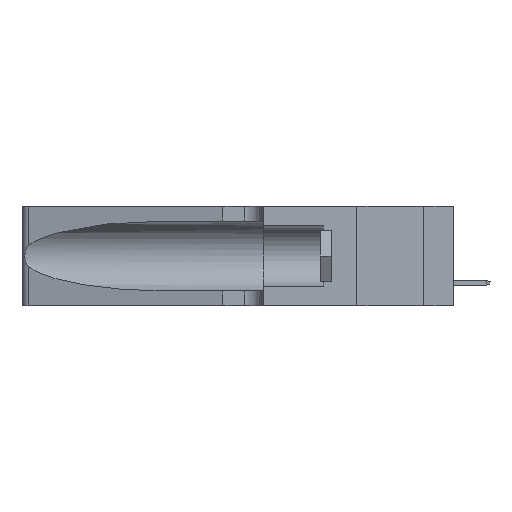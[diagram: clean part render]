
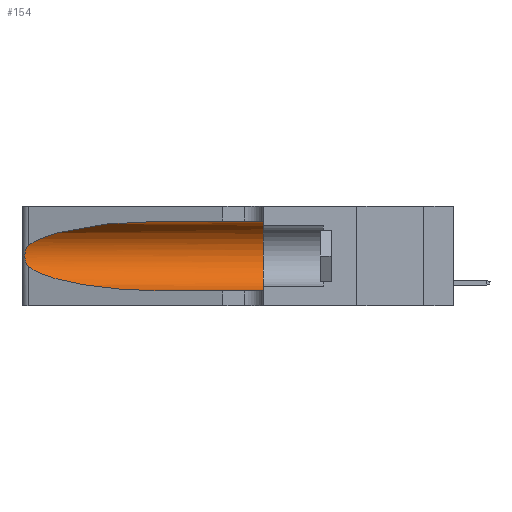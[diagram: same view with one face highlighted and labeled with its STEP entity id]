
A CAD part, left-side view. The second image highlights one B-rep face of the part: STEP entity #154.
In plain terms, the highlighted cylindrical face has radius 3.308 mm (diameter 6.617 mm), a partial arc.
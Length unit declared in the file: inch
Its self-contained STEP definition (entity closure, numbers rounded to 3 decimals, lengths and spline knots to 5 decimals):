
#131 = DIRECTION ( 'NONE',  ( 0., -1., 0. ) ) ;
#154 = ADVANCED_FACE ( 'NONE', ( #12733 ), #5379, .F. ) ;
#813 = ORIENTED_EDGE ( 'NONE', *, *, #28861, .T. ) ;
#963 = CARTESIAN_POINT ( 'NONE',  ( 0.25487, 1.22718, 0.14631 ) ) ;
#1753 = ORIENTED_EDGE ( 'NONE', *, *, #10633, .T. ) ;
#2669 = DIRECTION ( 'NONE',  ( 0., 0., 1. ) ) ;
#2769 = ORIENTED_EDGE ( 'NONE', *, *, #18886, .F. ) ;
#2884 = DIRECTION ( 'NONE',  ( 0., -1., 0. ) ) ;
#3205 = CARTESIAN_POINT ( 'NONE',  ( 0.25787, 1.23484, 0.2124 ) ) ;
#3506 = CARTESIAN_POINT ( 'NONE',  ( 0.25487, 1.22718, 0.22369 ) ) ;
#3818 = EDGE_CURVE ( 'NONE', #5532, #31102, #15495, .T. ) ;
#3832 = CARTESIAN_POINT ( 'NONE',  ( 0.25639, 1.23184, 0.21858 ) ) ;
#3978 = VERTEX_POINT ( 'NONE', #15798 ) ;
#4153 = VERTEX_POINT ( 'NONE', #15297 ) ;
#5379 = CYLINDRICAL_SURFACE ( 'NONE', #9538, 0.13025 ) ;
#5532 = VERTEX_POINT ( 'NONE', #25018 ) ;
#5560 = ORIENTED_EDGE ( 'NONE', *, *, #3818, .T. ) ;
#7277 = EDGE_CURVE ( 'NONE', #7630, #31102, #11832, .T. ) ;
#7630 = VERTEX_POINT ( 'NONE', #8875 ) ;
#8875 = CARTESIAN_POINT ( 'NONE',  ( 0.1305, 0.35, 0.31525 ) ) ;
#9178 = CARTESIAN_POINT ( 'NONE',  ( 0.1305, 0.72297, 0.31525 ) ) ;
#9538 = AXIS2_PLACEMENT_3D ( 'NONE', #10333, #131, #25272 ) ;
#9834 = CARTESIAN_POINT ( 'NONE',  ( 0.1305, 0.35, 0.05475 ) ) ;
#10003 =( BOUNDED_CURVE ( )  B_SPLINE_CURVE ( 3, ( #9178, #18931, #23084, #10980 ),
 .UNSPECIFIED., .F., .F. ) 
 B_SPLINE_CURVE_WITH_KNOTS ( ( 4, 4 ),
 ( 1.5708, 2.84003 ),
 .UNSPECIFIED. ) 
 CURVE ( )  GEOMETRIC_REPRESENTATION_ITEM ( )  RATIONAL_B_SPLINE_CURVE ( ( 1., 0.87, 0.87, 1. ) ) 
 REPRESENTATION_ITEM ( '' )  );
#10169 = CARTESIAN_POINT ( 'NONE',  ( 0.1305, 0.35, 0.185 ) ) ;
#10333 = CARTESIAN_POINT ( 'NONE',  ( 0.1305, 1.61858, 0.185 ) ) ;
#10548 = CARTESIAN_POINT ( 'NONE',  ( 0.26018, 1.23835, 0.19895 ) ) ;
#10633 = EDGE_CURVE ( 'NONE', #3978, #4153, #10003, .T. ) ;
#10980 = CARTESIAN_POINT ( 'NONE',  ( 0.25487, 1.22718, 0.22369 ) ) ;
#11832 = CIRCLE ( 'NONE', #26091, 0.13025 ) ;
#11880 =( BOUNDED_CURVE ( )  B_SPLINE_CURVE ( 3, ( #16994, #21289, #14752, #31005 ),
 .UNSPECIFIED., .F., .F. ) 
 B_SPLINE_CURVE_WITH_KNOTS ( ( 4, 4 ),
 ( 3.44316, 4.71239 ),
 .UNSPECIFIED. ) 
 CURVE ( )  GEOMETRIC_REPRESENTATION_ITEM ( )  RATIONAL_B_SPLINE_CURVE ( ( 1., 0.87, 0.87, 1. ) ) 
 REPRESENTATION_ITEM ( '' )  );
#12733 = FACE_OUTER_BOUND ( 'NONE', #21869, .T. ) ;
#14416 = CARTESIAN_POINT ( 'NONE',  ( 0.1305, 1.61858, 0.31525 ) ) ;
#14752 = CARTESIAN_POINT ( 'NONE',  ( 0.18966, 0.96281, 0.05475 ) ) ;
#15004 = VERTEX_POINT ( 'NONE', #24596 ) ;
#15297 = CARTESIAN_POINT ( 'NONE',  ( 0.25487, 1.22718, 0.22369 ) ) ;
#15495 = LINE ( 'NONE', #25210, #24383 ) ;
#15648 = CARTESIAN_POINT ( 'NONE',  ( 0.26075, 1.23896, 0.19203 ) ) ;
#15798 = CARTESIAN_POINT ( 'NONE',  ( 0.1305, 0.72297, 0.31525 ) ) ;
#15803 = EDGE_CURVE ( 'NONE', #15004, #5532, #11880, .T. ) ;
#16994 = CARTESIAN_POINT ( 'NONE',  ( 0.25487, 1.22718, 0.14631 ) ) ;
#18886 = EDGE_CURVE ( 'NONE', #3978, #7630, #26689, .T. ) ;
#18931 = CARTESIAN_POINT ( 'NONE',  ( 0.18966, 0.96281, 0.31525 ) ) ;
#20416 = CARTESIAN_POINT ( 'NONE',  ( 0.25639, 1.23186, 0.15144 ) ) ;
#20584 = CARTESIAN_POINT ( 'NONE',  ( 0.26075, 1.23896, 0.178 ) ) ;
#21111 = ORIENTED_EDGE ( 'NONE', *, *, #7277, .F. ) ;
#21289 = CARTESIAN_POINT ( 'NONE',  ( 0.2373, 1.15595, 0.08982 ) ) ;
#21517 = ORIENTED_EDGE ( 'NONE', *, *, #15803, .T. ) ;
#21869 = EDGE_LOOP ( 'NONE', ( #1753, #813, #21517, #5560, #21111, #2769 ) ) ;
#22811 = CARTESIAN_POINT ( 'NONE',  ( 0.25854, 1.2359, 0.20912 ) ) ;
#22967 = CARTESIAN_POINT ( 'NONE',  ( 0.25555, 1.22994, 0.2215 ) ) ;
#23084 = CARTESIAN_POINT ( 'NONE',  ( 0.2373, 1.15595, 0.28018 ) ) ;
#24383 = VECTOR ( 'NONE', #2884, 39.37008 ) ;
#24596 = CARTESIAN_POINT ( 'NONE',  ( 0.25487, 1.22718, 0.14631 ) ) ;
#25018 = CARTESIAN_POINT ( 'NONE',  ( 0.1305, 0.72297, 0.05475 ) ) ;
#25056 = CARTESIAN_POINT ( 'NONE',  ( 0.26017, 1.23833, 0.17102 ) ) ;
#25210 = CARTESIAN_POINT ( 'NONE',  ( 0.1305, 1.61858, 0.05475 ) ) ;
#25272 = DIRECTION ( 'NONE',  ( 0., 0., -1. ) ) ;
#25360 = CARTESIAN_POINT ( 'NONE',  ( 0.25856, 1.23593, 0.16098 ) ) ;
#26091 = AXIS2_PLACEMENT_3D ( 'NONE', #10169, #27389, #2669 ) ;
#26219 = DIRECTION ( 'NONE',  ( 0., -1., 0. ) ) ;
#26689 = LINE ( 'NONE', #14416, #30473 ) ;
#26764 = B_SPLINE_CURVE_WITH_KNOTS ( 'NONE', 3,
 ( #3506, #22967, #3832, #3205, #22811, #10548, #15648, #20584, #25056, #25360, #27924, #20416, #30464, #963 ),
 .UNSPECIFIED., .F., .F.,
 ( 4, 2, 2, 2, 2, 2, 4 ),
 ( 0., 0.00027, 0.00053, 0.00107, 0.0016, 0.00187, 0.00214 ),
 .UNSPECIFIED. ) ;
#27389 = DIRECTION ( 'NONE',  ( 0., 1., 0. ) ) ;
#27924 = CARTESIAN_POINT ( 'NONE',  ( 0.25789, 1.23486, 0.15765 ) ) ;
#28861 = EDGE_CURVE ( 'NONE', #4153, #15004, #26764, .T. ) ;
#30464 = CARTESIAN_POINT ( 'NONE',  ( 0.25555, 1.22993, 0.14849 ) ) ;
#30473 = VECTOR ( 'NONE', #26219, 39.37008 ) ;
#31005 = CARTESIAN_POINT ( 'NONE',  ( 0.1305, 0.72297, 0.05475 ) ) ;
#31102 = VERTEX_POINT ( 'NONE', #9834 ) ;
